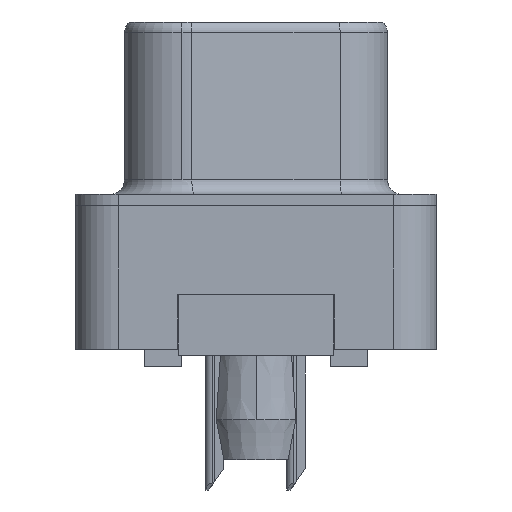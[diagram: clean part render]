
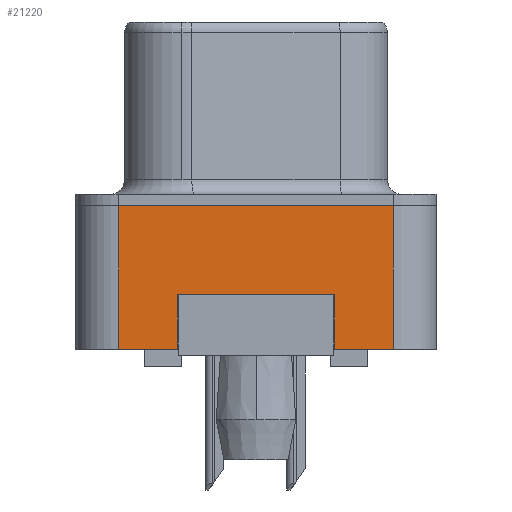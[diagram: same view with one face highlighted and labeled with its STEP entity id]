
A CAD part, left-side view. The second image highlights one B-rep face of the part: STEP entity #21220.
In plain terms, the highlighted planar face has unit normal (-1, 0, 0).
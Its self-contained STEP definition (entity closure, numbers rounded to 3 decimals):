
#28 = DIRECTION ( 'NONE',  ( 0., -1., 0. ) ) ;
#35 = DIRECTION ( 'NONE',  ( 0., 0., -1. ) ) ;
#528 = LINE ( 'NONE', #22363, #6702 ) ;
#634 = VERTEX_POINT ( 'NONE', #3894 ) ;
#712 = ORIENTED_EDGE ( 'NONE', *, *, #13348, .F. ) ;
#1070 = EDGE_CURVE ( 'NONE', #16143, #5355, #3627, .T. ) ;
#1342 = VECTOR ( 'NONE', #17068, 1000. ) ;
#1760 = VECTOR ( 'NONE', #13238, 1000. ) ;
#1990 = VECTOR ( 'NONE', #13617, 1000. ) ;
#2197 = ORIENTED_EDGE ( 'NONE', *, *, #7354, .T. ) ;
#2228 = EDGE_LOOP ( 'NONE', ( #18182, #2197, #6157, #4106, #9111, #10471, #712, #6194 ) ) ;
#2568 = LINE ( 'NONE', #2685, #1990 ) ;
#2572 = CARTESIAN_POINT ( 'NONE',  ( -3., -4.775, -5. ) ) ;
#2685 = CARTESIAN_POINT ( 'NONE',  ( -3., -2.75, -3.1 ) ) ;
#3627 = LINE ( 'NONE', #16231, #5592 ) ;
#3742 = VECTOR ( 'NONE', #10791, 1000. ) ;
#3894 = CARTESIAN_POINT ( 'NONE',  ( -3., -4.775, -5. ) ) ;
#4106 = ORIENTED_EDGE ( 'NONE', *, *, #1070, .F. ) ;
#4276 = DIRECTION ( 'NONE',  ( 0., 0., 1. ) ) ;
#4568 = LINE ( 'NONE', #20852, #1760 ) ;
#4643 = VECTOR ( 'NONE', #28, 1000. ) ;
#4802 = EDGE_CURVE ( 'NONE', #10884, #16143, #23282, .T. ) ;
#5176 = CARTESIAN_POINT ( 'NONE',  ( -3., 4.775, 0. ) ) ;
#5355 = VERTEX_POINT ( 'NONE', #22851 ) ;
#5473 = LINE ( 'NONE', #21283, #4643 ) ;
#5592 = VECTOR ( 'NONE', #10974, 1000. ) ;
#5685 = CARTESIAN_POINT ( 'NONE',  ( -3., 4.775, -5. ) ) ;
#6157 = ORIENTED_EDGE ( 'NONE', *, *, #10998, .T. ) ;
#6194 = ORIENTED_EDGE ( 'NONE', *, *, #13025, .F. ) ;
#6702 = VECTOR ( 'NONE', #16900, 1000. ) ;
#7354 = EDGE_CURVE ( 'NONE', #9682, #634, #5473, .T. ) ;
#7672 = CARTESIAN_POINT ( 'NONE',  ( -3., 2.75, -3.1 ) ) ;
#9022 = LINE ( 'NONE', #21525, #21140 ) ;
#9111 = ORIENTED_EDGE ( 'NONE', *, *, #4802, .F. ) ;
#9682 = VERTEX_POINT ( 'NONE', #20390 ) ;
#10471 = ORIENTED_EDGE ( 'NONE', *, *, #12590, .T. ) ;
#10791 = DIRECTION ( 'NONE',  ( 0., 0., 1. ) ) ;
#10884 = VERTEX_POINT ( 'NONE', #14343 ) ;
#10974 = DIRECTION ( 'NONE',  ( 0., -1., 0. ) ) ;
#10998 = EDGE_CURVE ( 'NONE', #634, #5355, #11833, .T. ) ;
#11833 = LINE ( 'NONE', #2572, #1342 ) ;
#12051 = CARTESIAN_POINT ( 'NONE',  ( -3., -2.75, -3.1 ) ) ;
#12590 = EDGE_CURVE ( 'NONE', #10884, #16220, #4568, .T. ) ;
#13025 = EDGE_CURVE ( 'NONE', #15178, #23273, #528, .T. ) ;
#13238 = DIRECTION ( 'NONE',  ( 0., -1., 0. ) ) ;
#13348 = EDGE_CURVE ( 'NONE', #23273, #16220, #9022, .T. ) ;
#13617 = DIRECTION ( 'NONE',  ( 0., 0., -1. ) ) ;
#14343 = CARTESIAN_POINT ( 'NONE',  ( -3., 4.775, -5. ) ) ;
#15178 = VERTEX_POINT ( 'NONE', #12051 ) ;
#16143 = VERTEX_POINT ( 'NONE', #5176 ) ;
#16220 = VERTEX_POINT ( 'NONE', #23108 ) ;
#16231 = CARTESIAN_POINT ( 'NONE',  ( -3., -4.775, 0. ) ) ;
#16454 = AXIS2_PLACEMENT_3D ( 'NONE', #19011, #22696, #4276 ) ;
#16900 = DIRECTION ( 'NONE',  ( 0., 1., 0. ) ) ;
#17068 = DIRECTION ( 'NONE',  ( 0., 0., 1. ) ) ;
#18182 = ORIENTED_EDGE ( 'NONE', *, *, #23363, .T. ) ;
#19011 = CARTESIAN_POINT ( 'NONE',  ( -3., -4.775, -5. ) ) ;
#20390 = CARTESIAN_POINT ( 'NONE',  ( -3., -2.75, -5. ) ) ;
#20560 = FACE_OUTER_BOUND ( 'NONE', #2228, .T. ) ;
#20852 = CARTESIAN_POINT ( 'NONE',  ( -3., -4.775, -5. ) ) ;
#21140 = VECTOR ( 'NONE', #35, 1000. ) ;
#21220 = ADVANCED_FACE ( 'NONE', ( #20560 ), #22452, .T. ) ;
#21283 = CARTESIAN_POINT ( 'NONE',  ( -3., -4.775, -5. ) ) ;
#21525 = CARTESIAN_POINT ( 'NONE',  ( -3., 2.75, -3.1 ) ) ;
#22363 = CARTESIAN_POINT ( 'NONE',  ( -3., 2.75, -3.1 ) ) ;
#22452 = PLANE ( 'NONE',  #16454 ) ;
#22696 = DIRECTION ( 'NONE',  ( -1., 0., 0. ) ) ;
#22851 = CARTESIAN_POINT ( 'NONE',  ( -3., -4.775, 0. ) ) ;
#23108 = CARTESIAN_POINT ( 'NONE',  ( -3., 2.75, -5. ) ) ;
#23273 = VERTEX_POINT ( 'NONE', #7672 ) ;
#23282 = LINE ( 'NONE', #5685, #3742 ) ;
#23363 = EDGE_CURVE ( 'NONE', #15178, #9682, #2568, .T. ) ;
